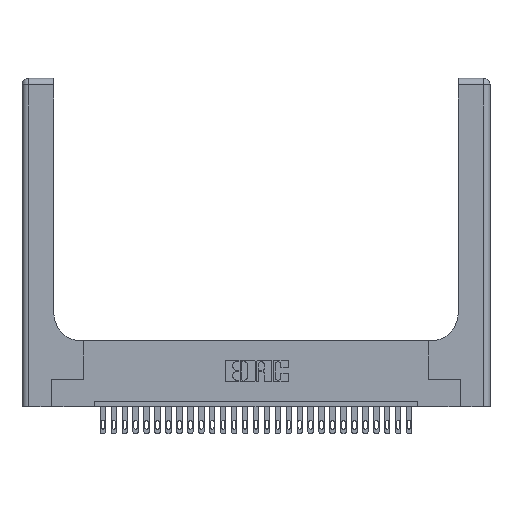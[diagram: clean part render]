
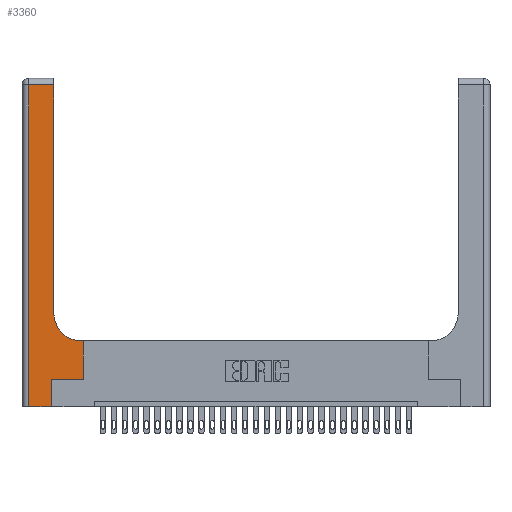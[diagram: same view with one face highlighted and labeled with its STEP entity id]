
A CAD part, top view. The second image highlights one B-rep face of the part: STEP entity #3360.
In plain terms, the highlighted planar face has unit normal (0, 0, 1).
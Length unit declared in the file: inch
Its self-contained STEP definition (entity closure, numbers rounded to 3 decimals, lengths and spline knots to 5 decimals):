
#205 = CARTESIAN_POINT ( 'NONE',  ( 0.2915, 2.94, 0.37 ) ) ;
#372 = ORIENTED_EDGE ( 'NONE', *, *, #17894, .T. ) ;
#435 = LINE ( 'NONE', #19001, #9418 ) ;
#700 = EDGE_CURVE ( 'NONE', #12751, #8036, #2388, .T. ) ;
#1083 = CARTESIAN_POINT ( 'NONE',  ( 0.5585, 0.25, 0.37 ) ) ;
#1549 = VERTEX_POINT ( 'NONE', #2640 ) ;
#2388 = LINE ( 'NONE', #19157, #19350 ) ;
#2423 = VERTEX_POINT ( 'NONE', #11544 ) ;
#2640 = CARTESIAN_POINT ( 'NONE',  ( 0.269, 0., 0.37 ) ) ;
#2821 = ORIENTED_EDGE ( 'NONE', *, *, #28147, .T. ) ;
#2946 = CARTESIAN_POINT ( 'NONE',  ( 0.5415, 0.85, 0.37 ) ) ;
#3360 = ADVANCED_FACE ( 'NONE', ( #16655 ), #17218, .F. ) ;
#3722 = DIRECTION ( 'NONE',  ( 0., 1., 0. ) ) ;
#4276 = AXIS2_PLACEMENT_3D ( 'NONE', #2946, #27441, #27347 ) ;
#4490 = VERTEX_POINT ( 'NONE', #12594 ) ;
#4979 = ORIENTED_EDGE ( 'NONE', *, *, #27263, .T. ) ;
#6542 = CIRCLE ( 'NONE', #4276, 0.25 ) ;
#6806 = VECTOR ( 'NONE', #13628, 39.37008 ) ;
#6910 = ORIENTED_EDGE ( 'NONE', *, *, #16194, .T. ) ;
#7025 = EDGE_CURVE ( 'NONE', #1549, #2423, #8490, .T. ) ;
#7199 = VECTOR ( 'NONE', #11962, 39.37008 ) ;
#8036 = VERTEX_POINT ( 'NONE', #25722 ) ;
#8490 = LINE ( 'NONE', #14543, #16838 ) ;
#8569 = LINE ( 'NONE', #21480, #23119 ) ;
#8743 = EDGE_CURVE ( 'NONE', #14591, #1549, #435, .T. ) ;
#9418 = VECTOR ( 'NONE', #21009, 39.37008 ) ;
#10091 = VERTEX_POINT ( 'NONE', #205 ) ;
#11544 = CARTESIAN_POINT ( 'NONE',  ( 0.269, 0.25, 0.37 ) ) ;
#11590 = DIRECTION ( 'NONE',  ( -1., 0., 0. ) ) ;
#11895 = EDGE_CURVE ( 'NONE', #21228, #10091, #24941, .T. ) ;
#11962 = DIRECTION ( 'NONE',  ( 0., 1., 0. ) ) ;
#12594 = CARTESIAN_POINT ( 'NONE',  ( 0.06, 2.94, 0.37 ) ) ;
#12751 = VERTEX_POINT ( 'NONE', #27752 ) ;
#12944 = LINE ( 'NONE', #21356, #19532 ) ;
#13027 = CARTESIAN_POINT ( 'NONE',  ( 0.2915, 0.85, 0.37 ) ) ;
#13628 = DIRECTION ( 'NONE',  ( 0., -1., 0. ) ) ;
#14171 = CARTESIAN_POINT ( 'NONE',  ( 0.06, 0., 0.37 ) ) ;
#14234 = ORIENTED_EDGE ( 'NONE', *, *, #23838, .T. ) ;
#14543 = CARTESIAN_POINT ( 'NONE',  ( 0.269, 0., 0.37 ) ) ;
#14591 = VERTEX_POINT ( 'NONE', #14171 ) ;
#15146 = CARTESIAN_POINT ( 'NONE',  ( 0.06, 3., 0.37 ) ) ;
#15217 = DIRECTION ( 'NONE',  ( -1., 0., 0. ) ) ;
#15229 = ORIENTED_EDGE ( 'NONE', *, *, #8743, .T. ) ;
#16194 = EDGE_CURVE ( 'NONE', #8036, #21228, #6542, .T. ) ;
#16655 = FACE_OUTER_BOUND ( 'NONE', #27372, .T. ) ;
#16838 = VECTOR ( 'NONE', #28202, 39.37008 ) ;
#17218 = PLANE ( 'NONE',  #25006 ) ;
#17894 = EDGE_CURVE ( 'NONE', #4490, #14591, #21022, .T. ) ;
#19001 = CARTESIAN_POINT ( 'NONE',  ( 0., 0., 0.37 ) ) ;
#19060 = VECTOR ( 'NONE', #3722, 39.37008 ) ;
#19157 = CARTESIAN_POINT ( 'NONE',  ( 0.2915, 0.6, 0.37 ) ) ;
#19350 = VECTOR ( 'NONE', #28572, 39.37008 ) ;
#19438 = CARTESIAN_POINT ( 'NONE',  ( 0.2915, 3., 0.37 ) ) ;
#19490 = ORIENTED_EDGE ( 'NONE', *, *, #11895, .T. ) ;
#19532 = VECTOR ( 'NONE', #11590, 39.37008 ) ;
#19645 = CARTESIAN_POINT ( 'NONE',  ( 0., 3., 0.37 ) ) ;
#21009 = DIRECTION ( 'NONE',  ( 1., 0., 0. ) ) ;
#21022 = LINE ( 'NONE', #15146, #6806 ) ;
#21228 = VERTEX_POINT ( 'NONE', #13027 ) ;
#21356 = CARTESIAN_POINT ( 'NONE',  ( 0., 2.94, 0.37 ) ) ;
#21480 = CARTESIAN_POINT ( 'NONE',  ( 0.269, 0.25, 0.37 ) ) ;
#22140 = ORIENTED_EDGE ( 'NONE', *, *, #700, .T. ) ;
#23119 = VECTOR ( 'NONE', #27988, 39.37008 ) ;
#23838 = EDGE_CURVE ( 'NONE', #10091, #4490, #12944, .T. ) ;
#24680 = CARTESIAN_POINT ( 'NONE',  ( 0.5585, 0.25, 0.37 ) ) ;
#24941 = LINE ( 'NONE', #19438, #19060 ) ;
#25006 = AXIS2_PLACEMENT_3D ( 'NONE', #19645, #26247, #15217 ) ;
#25340 = VERTEX_POINT ( 'NONE', #24680 ) ;
#25722 = CARTESIAN_POINT ( 'NONE',  ( 0.5415, 0.6, 0.37 ) ) ;
#26247 = DIRECTION ( 'NONE',  ( 0., 0., -1. ) ) ;
#27263 = EDGE_CURVE ( 'NONE', #25340, #12751, #28040, .T. ) ;
#27347 = DIRECTION ( 'NONE',  ( 1., 0., 0. ) ) ;
#27372 = EDGE_LOOP ( 'NONE', ( #19490, #14234, #372, #15229, #27432, #2821, #4979, #22140, #6910 ) ) ;
#27432 = ORIENTED_EDGE ( 'NONE', *, *, #7025, .T. ) ;
#27441 = DIRECTION ( 'NONE',  ( 0., 0., -1. ) ) ;
#27752 = CARTESIAN_POINT ( 'NONE',  ( 0.5585, 0.6, 0.37 ) ) ;
#27988 = DIRECTION ( 'NONE',  ( 1., 0., 0. ) ) ;
#28040 = LINE ( 'NONE', #1083, #7199 ) ;
#28147 = EDGE_CURVE ( 'NONE', #2423, #25340, #8569, .T. ) ;
#28202 = DIRECTION ( 'NONE',  ( 0., 1., 0. ) ) ;
#28572 = DIRECTION ( 'NONE',  ( -1., 0., 0. ) ) ;
